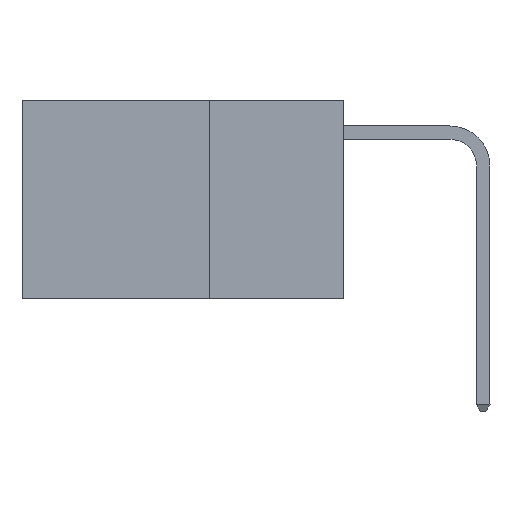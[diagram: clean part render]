
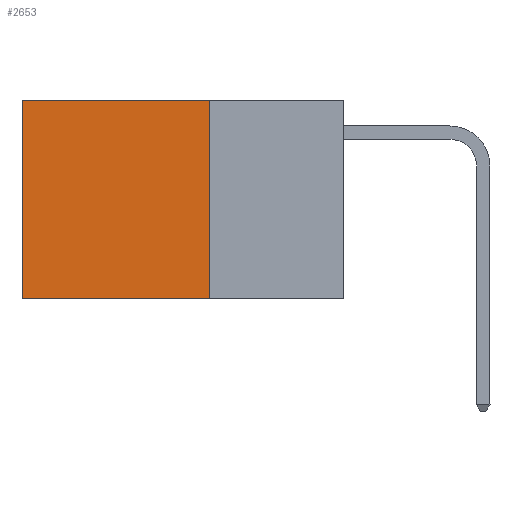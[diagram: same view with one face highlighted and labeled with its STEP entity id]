
A CAD part, left-side view. The second image highlights one B-rep face of the part: STEP entity #2653.
In plain terms, the highlighted planar face has unit normal (-1, 0, 0).
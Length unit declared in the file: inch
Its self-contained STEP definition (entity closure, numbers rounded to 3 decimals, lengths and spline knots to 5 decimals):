
#91 = VERTEX_POINT ( 'NONE', #9303 ) ;
#328 = VERTEX_POINT ( 'NONE', #4059 ) ;
#468 = EDGE_CURVE ( 'NONE', #328, #91, #4103, .T. ) ;
#469 = VECTOR ( 'NONE', #3782, 39.37008 ) ;
#552 = VECTOR ( 'NONE', #9247, 39.37008 ) ;
#1582 = DIRECTION ( 'NONE',  ( 0., 1., 0. ) ) ;
#1681 = CARTESIAN_POINT ( 'NONE',  ( 0.2625, 0.25, -0.37 ) ) ;
#1728 = LINE ( 'NONE', #13831, #469 ) ;
#2283 = FACE_OUTER_BOUND ( 'NONE', #7448, .T. ) ;
#2653 = ADVANCED_FACE ( 'NONE', ( #2283 ), #15174, .F. ) ;
#2704 = VECTOR ( 'NONE', #1582, 39.37008 ) ;
#2729 = ORIENTED_EDGE ( 'NONE', *, *, #3853, .F. ) ;
#3331 = VERTEX_POINT ( 'NONE', #6650 ) ;
#3674 = EDGE_CURVE ( 'NONE', #3331, #10754, #6241, .T. ) ;
#3778 = DIRECTION ( 'NONE',  ( 0., 0., -1. ) ) ;
#3782 = DIRECTION ( 'NONE',  ( 0., 0., -1. ) ) ;
#3853 = EDGE_CURVE ( 'NONE', #328, #3331, #10314, .T. ) ;
#4059 = CARTESIAN_POINT ( 'NONE',  ( 0.2625, 0.25, 0. ) ) ;
#4103 = LINE ( 'NONE', #14086, #552 ) ;
#6241 = LINE ( 'NONE', #1681, #2704 ) ;
#6650 = CARTESIAN_POINT ( 'NONE',  ( 0.2625, 0.25, -0.37 ) ) ;
#7448 = EDGE_LOOP ( 'NONE', ( #10924, #11962, #2729, #13727 ) ) ;
#8086 = CARTESIAN_POINT ( 'NONE',  ( 0.2625, 0.6, -0.37 ) ) ;
#8087 = CARTESIAN_POINT ( 'NONE',  ( 0.2625, 0.25, 0. ) ) ;
#9247 = DIRECTION ( 'NONE',  ( 0., 1., 0. ) ) ;
#9303 = CARTESIAN_POINT ( 'NONE',  ( 0.2625, 0.6, 0. ) ) ;
#10314 = LINE ( 'NONE', #8087, #13194 ) ;
#10754 = VERTEX_POINT ( 'NONE', #8086 ) ;
#10924 = ORIENTED_EDGE ( 'NONE', *, *, #15613, .T. ) ;
#11962 = ORIENTED_EDGE ( 'NONE', *, *, #3674, .F. ) ;
#13194 = VECTOR ( 'NONE', #3778, 39.37008 ) ;
#13727 = ORIENTED_EDGE ( 'NONE', *, *, #468, .T. ) ;
#13831 = CARTESIAN_POINT ( 'NONE',  ( 0.2625, 0.6, 0. ) ) ;
#14086 = CARTESIAN_POINT ( 'NONE',  ( 0.2625, 0.25, 0. ) ) ;
#14440 = AXIS2_PLACEMENT_3D ( 'NONE', #15733, #15151, #15121 ) ;
#15121 = DIRECTION ( 'NONE',  ( 0., 0., -1. ) ) ;
#15151 = DIRECTION ( 'NONE',  ( 1., 0., 0. ) ) ;
#15174 = PLANE ( 'NONE',  #14440 ) ;
#15613 = EDGE_CURVE ( 'NONE', #91, #10754, #1728, .T. ) ;
#15733 = CARTESIAN_POINT ( 'NONE',  ( 0.2625, 0.25, 0. ) ) ;
